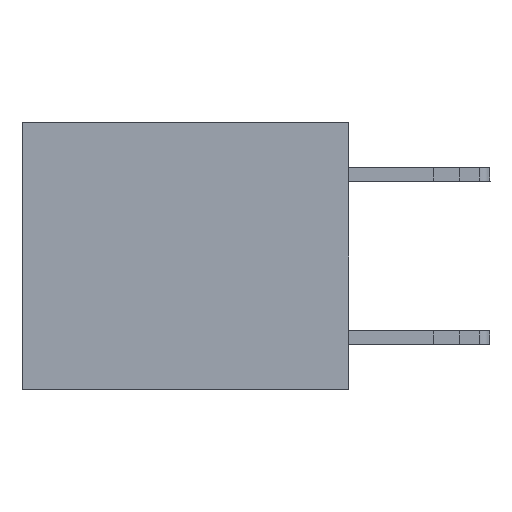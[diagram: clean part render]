
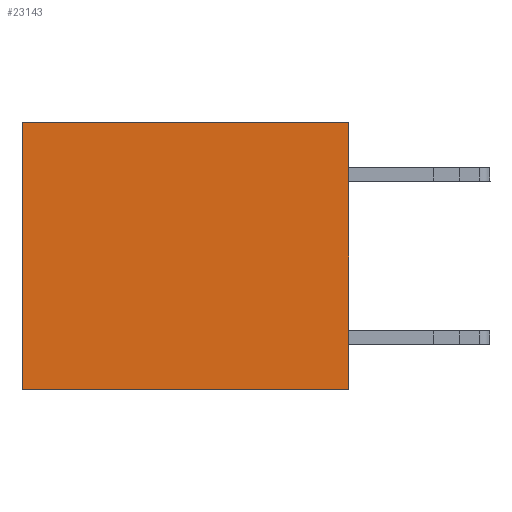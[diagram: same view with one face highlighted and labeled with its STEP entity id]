
A CAD part, left-side view. The second image highlights one B-rep face of the part: STEP entity #23143.
In plain terms, the highlighted planar face has unit normal (-1, 0, 0).
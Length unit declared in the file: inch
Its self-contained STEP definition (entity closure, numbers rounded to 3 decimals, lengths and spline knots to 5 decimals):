
#174 = EDGE_CURVE ( 'NONE', #9954, #29855, #9580, .T. ) ;
#253 = ORIENTED_EDGE ( 'NONE', *, *, #10620, .T. ) ;
#1224 = CARTESIAN_POINT ( 'NONE',  ( 0.3165, 0., -0.49 ) ) ;
#1332 = DIRECTION ( 'NONE',  ( 0., 1., 0. ) ) ;
#1982 = DIRECTION ( 'NONE',  ( 0., 0., -1. ) ) ;
#4556 = CARTESIAN_POINT ( 'NONE',  ( 0.3165, 0., -0.49 ) ) ;
#6008 = EDGE_CURVE ( 'NONE', #9954, #19678, #16131, .T. ) ;
#8885 = EDGE_CURVE ( 'NONE', #29855, #14343, #15115, .T. ) ;
#9126 = ORIENTED_EDGE ( 'NONE', *, *, #8885, .F. ) ;
#9580 = LINE ( 'NONE', #18201, #11582 ) ;
#9769 = PLANE ( 'NONE',  #21042 ) ;
#9954 = VERTEX_POINT ( 'NONE', #28268 ) ;
#10620 = EDGE_CURVE ( 'NONE', #19678, #14343, #27333, .T. ) ;
#10724 = CARTESIAN_POINT ( 'NONE',  ( 0.3165, 0.6, -0.49 ) ) ;
#11387 = EDGE_LOOP ( 'NONE', ( #253, #9126, #19166, #20717 ) ) ;
#11582 = VECTOR ( 'NONE', #25945, 39.37008 ) ;
#14343 = VERTEX_POINT ( 'NONE', #18683 ) ;
#15115 = LINE ( 'NONE', #32181, #30437 ) ;
#15720 = VECTOR ( 'NONE', #32295, 39.37008 ) ;
#16131 = LINE ( 'NONE', #24864, #15720 ) ;
#18201 = CARTESIAN_POINT ( 'NONE',  ( 0.3165, 0., -0.49 ) ) ;
#18683 = CARTESIAN_POINT ( 'NONE',  ( 0.3165, 0.6, -0.49 ) ) ;
#19166 = ORIENTED_EDGE ( 'NONE', *, *, #174, .F. ) ;
#19678 = VERTEX_POINT ( 'NONE', #29978 ) ;
#19975 = DIRECTION ( 'NONE',  ( 1., 0., 0. ) ) ;
#20717 = ORIENTED_EDGE ( 'NONE', *, *, #6008, .T. ) ;
#21042 = AXIS2_PLACEMENT_3D ( 'NONE', #4556, #19975, #1982 ) ;
#23143 = ADVANCED_FACE ( 'NONE', ( #25886 ), #9769, .F. ) ;
#24864 = CARTESIAN_POINT ( 'NONE',  ( 0.3165, 0., 0. ) ) ;
#25886 = FACE_OUTER_BOUND ( 'NONE', #11387, .T. ) ;
#25945 = DIRECTION ( 'NONE',  ( 0., 0., -1. ) ) ;
#27333 = LINE ( 'NONE', #10724, #29327 ) ;
#28268 = CARTESIAN_POINT ( 'NONE',  ( 0.3165, 0., 0. ) ) ;
#29327 = VECTOR ( 'NONE', #31466, 39.37008 ) ;
#29855 = VERTEX_POINT ( 'NONE', #1224 ) ;
#29978 = CARTESIAN_POINT ( 'NONE',  ( 0.3165, 0.6, 0. ) ) ;
#30437 = VECTOR ( 'NONE', #1332, 39.37008 ) ;
#31466 = DIRECTION ( 'NONE',  ( 0., 0., -1. ) ) ;
#32181 = CARTESIAN_POINT ( 'NONE',  ( 0.3165, 0., -0.49 ) ) ;
#32295 = DIRECTION ( 'NONE',  ( 0., 1., 0. ) ) ;
